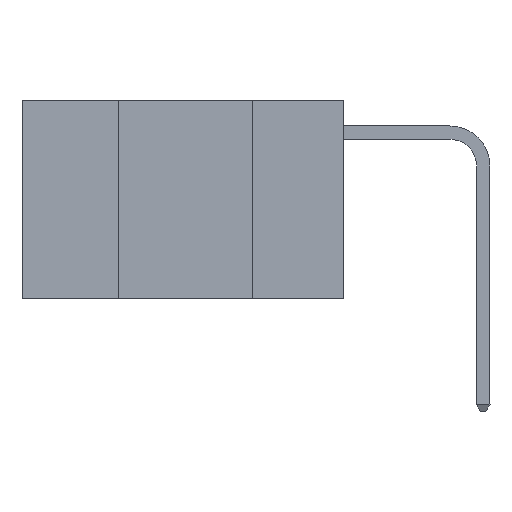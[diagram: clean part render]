
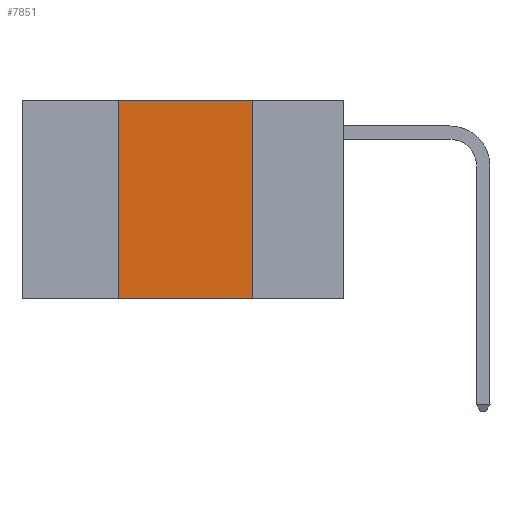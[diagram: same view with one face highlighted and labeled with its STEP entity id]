
A CAD part, left-side view. The second image highlights one B-rep face of the part: STEP entity #7851.
In plain terms, the highlighted planar face has unit normal (-1, 0, 0).
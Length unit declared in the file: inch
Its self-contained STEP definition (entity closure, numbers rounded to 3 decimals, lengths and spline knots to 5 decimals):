
#148 = CARTESIAN_POINT ( 'NONE',  ( 0., 0.17, 0. ) ) ;
#294 = CARTESIAN_POINT ( 'NONE',  ( 0., 0.6, 0. ) ) ;
#340 = PLANE ( 'NONE',  #1420 ) ;
#573 = VECTOR ( 'NONE', #1888, 39.37008 ) ;
#581 = LINE ( 'NONE', #1933, #573 ) ;
#1041 = VERTEX_POINT ( 'NONE', #11454 ) ;
#1420 = AXIS2_PLACEMENT_3D ( 'NONE', #294, #11474, #11996 ) ;
#1668 = EDGE_CURVE ( 'NONE', #2073, #3430, #5476, .T. ) ;
#1888 = DIRECTION ( 'NONE',  ( 0., -1., 0. ) ) ;
#1933 = CARTESIAN_POINT ( 'NONE',  ( 0., 0.6, 0. ) ) ;
#2073 = VERTEX_POINT ( 'NONE', #4112 ) ;
#2293 = VECTOR ( 'NONE', #4690, 39.37008 ) ;
#2544 = ORIENTED_EDGE ( 'NONE', *, *, #4620, .T. ) ;
#3430 = VERTEX_POINT ( 'NONE', #6147 ) ;
#3470 = VECTOR ( 'NONE', #5200, 39.37008 ) ;
#3810 = LINE ( 'NONE', #5348, #3470 ) ;
#4112 = CARTESIAN_POINT ( 'NONE',  ( 0., 0.17, 0. ) ) ;
#4120 = EDGE_CURVE ( 'NONE', #6201, #1041, #4560, .T. ) ;
#4268 = VECTOR ( 'NONE', #8414, 39.37008 ) ;
#4477 = ORIENTED_EDGE ( 'NONE', *, *, #1668, .F. ) ;
#4560 = LINE ( 'NONE', #8461, #4268 ) ;
#4620 = EDGE_CURVE ( 'NONE', #6201, #3430, #3810, .T. ) ;
#4690 = DIRECTION ( 'NONE',  ( 0., 0., -1. ) ) ;
#4980 = ORIENTED_EDGE ( 'NONE', *, *, #4120, .F. ) ;
#5019 = EDGE_CURVE ( 'NONE', #1041, #2073, #581, .T. ) ;
#5200 = DIRECTION ( 'NONE',  ( 0., -1., 0. ) ) ;
#5325 = ORIENTED_EDGE ( 'NONE', *, *, #5019, .F. ) ;
#5348 = CARTESIAN_POINT ( 'NONE',  ( 0., 0.6, -0.37 ) ) ;
#5476 = LINE ( 'NONE', #148, #2293 ) ;
#6147 = CARTESIAN_POINT ( 'NONE',  ( 0., 0.17, -0.37 ) ) ;
#6201 = VERTEX_POINT ( 'NONE', #8241 ) ;
#7012 = EDGE_LOOP ( 'NONE', ( #4477, #5325, #4980, #2544 ) ) ;
#7851 = ADVANCED_FACE ( 'NONE', ( #11602 ), #340, .F. ) ;
#8241 = CARTESIAN_POINT ( 'NONE',  ( 0., 0.42, -0.37 ) ) ;
#8414 = DIRECTION ( 'NONE',  ( 0., 0., 1. ) ) ;
#8461 = CARTESIAN_POINT ( 'NONE',  ( 0., 0.42, 0. ) ) ;
#11454 = CARTESIAN_POINT ( 'NONE',  ( 0., 0.42, 0. ) ) ;
#11474 = DIRECTION ( 'NONE',  ( 1., 0., 0. ) ) ;
#11602 = FACE_OUTER_BOUND ( 'NONE', #7012, .T. ) ;
#11996 = DIRECTION ( 'NONE',  ( 0., 0., -1. ) ) ;
